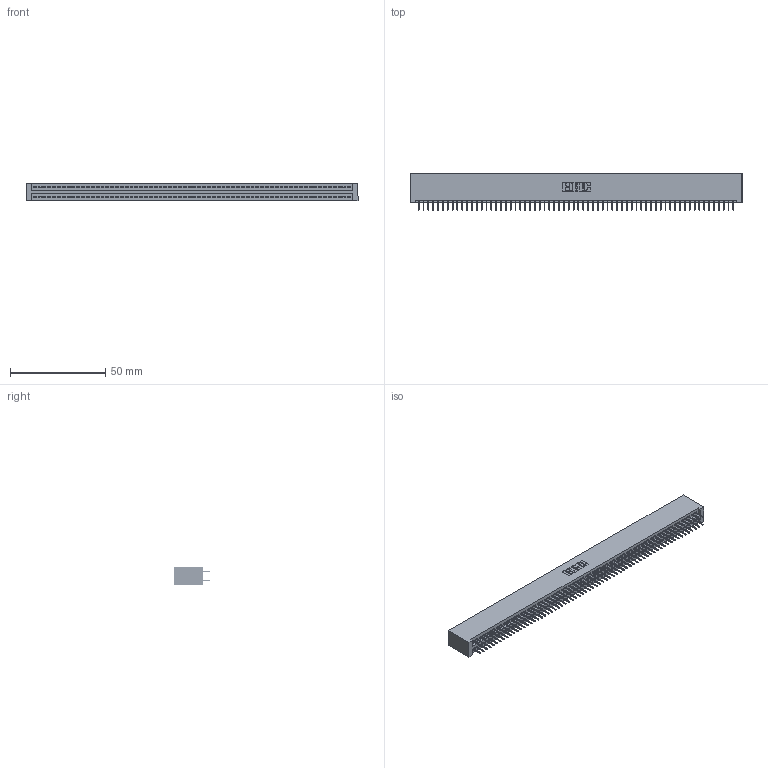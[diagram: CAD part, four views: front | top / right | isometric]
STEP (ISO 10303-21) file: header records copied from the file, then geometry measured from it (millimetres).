
FILE_DESCRIPTION (( 'STEP AP203' ), '1' );
FILE_NAME ('345-132-524-201.STEP', '2019-11-07T20:20:11', ( '' ), ( '' ), 'SwSTEP 2.0', 'SolidWorks 2016', '' );
FILE_SCHEMA (( 'CONFIG_CONTROL_DESIGN' ));
Length unit declared in the file: inch
Products named in the file (3): 345 Part_No Mounting Lugs; 345-292-001_345-293-124; 345-132-524-201
Assembly tree (133 placements, depth 2):
  345-132-524-201
    345 Part_No Mounting Lugs
    345-292-001_345-293-124  x132
Bounding box: 174.24 x 19.35 x 9.4 mm (x, y, z)
Volume: 17565.2 mm3; surface area: 26205 mm2
Topology: 133 solids, 133 shells, 7246 faces, 20513 edges, 13146 vertices
Faces by surface type: plane 5224, cylinder 2022
Entity records: 48351 total; most frequent: CARTESIAN_POINT 8080, ORIENTED_EDGE 8014, DIRECTION 7091, EDGE_CURVE 4007, LINE 3623, VECTOR 3623, VERTEX_POINT 2666, AXIS2_PLACEMENT_3D 1734
